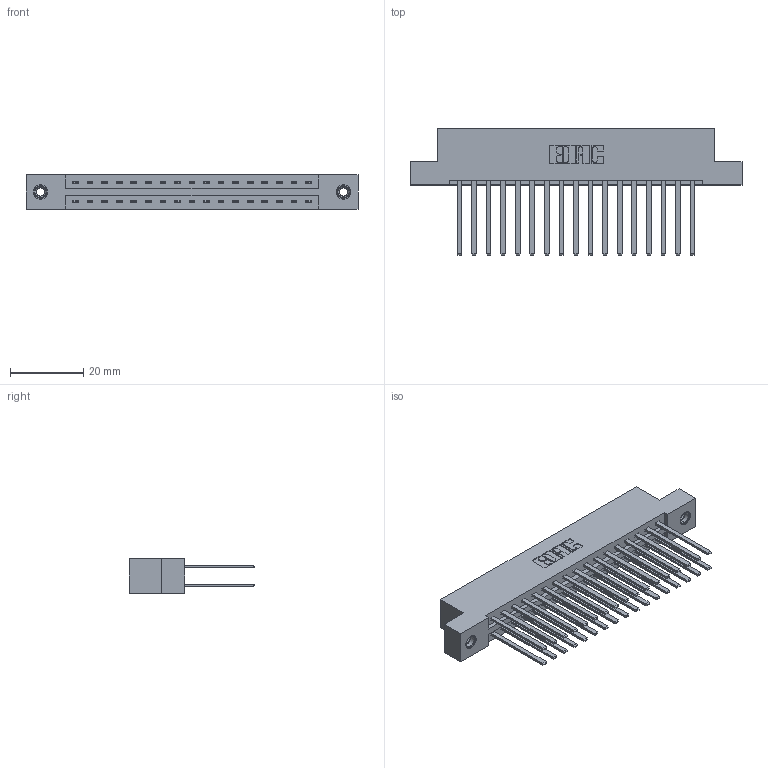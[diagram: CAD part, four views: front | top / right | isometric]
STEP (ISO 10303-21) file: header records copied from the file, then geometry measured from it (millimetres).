
FILE_DESCRIPTION (( 'STEP AP203' ), '1' );
FILE_NAME ('387-034-544-208.STEP', '2019-10-17T17:47:24', ( '' ), ( '' ), 'SwSTEP 2.0', 'SolidWorks 2016', '' );
FILE_SCHEMA (( 'CONFIG_CONTROL_DESIGN' ));
Length unit declared in the file: inch
Products named in the file (4): 337 Part_Flush Mounting Lugs - 0.156 Dia-TI; 345-292-001_345-293-144; 387-034-544-208; 345-250-001_345-250-003-102
Assembly tree (37 placements, depth 2):
  387-034-544-208
    337 Part_Flush Mounting Lugs - 0.156 Dia-TI
    345-292-001_345-293-144  x34
    345-250-001_345-250-003-102  x2
Bounding box: 90.37 x 34.3 x 9.4 mm (x, y, z)
Volume: 9661.6 mm3; surface area: 12260.5 mm2
Topology: 37 solids, 37 shells, 1806 faces, 5309 edges, 3486 vertices
Faces by surface type: plane 1258, cylinder 532, cone 12, torus 4
Entity records: 17416 total; most frequent: CARTESIAN_POINT 2933, ORIENTED_EDGE 2862, DIRECTION 2569, EDGE_CURVE 1431, LINE 1287, VECTOR 1287, VERTEX_POINT 948, AXIS2_PLACEMENT_3D 641
